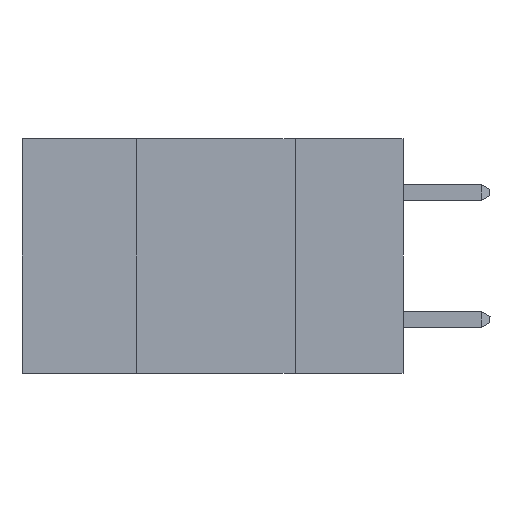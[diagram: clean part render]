
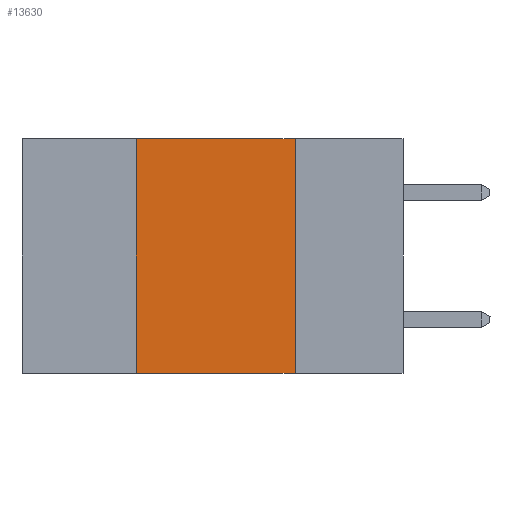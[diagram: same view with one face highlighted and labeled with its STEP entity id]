
A CAD part, left-side view. The second image highlights one B-rep face of the part: STEP entity #13630.
In plain terms, the highlighted planar face has unit normal (-1, 0, 0).
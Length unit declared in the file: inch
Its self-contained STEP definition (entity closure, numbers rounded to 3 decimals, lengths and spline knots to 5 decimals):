
#1485 = FACE_OUTER_BOUND ( 'NONE', #4667, .T. ) ;
#1644 = CARTESIAN_POINT ( 'NONE',  ( 0., 0.42, 0. ) ) ;
#1658 = CARTESIAN_POINT ( 'NONE',  ( 0., 0.6, -0.37 ) ) ;
#2081 = CARTESIAN_POINT ( 'NONE',  ( 0., 0.42, -0.37 ) ) ;
#2156 = EDGE_CURVE ( 'NONE', #14228, #9440, #12163, .T. ) ;
#3195 = VERTEX_POINT ( 'NONE', #16575 ) ;
#4179 = ORIENTED_EDGE ( 'NONE', *, *, #10590, .F. ) ;
#4345 = DIRECTION ( 'NONE',  ( 0., -1., 0. ) ) ;
#4667 = EDGE_LOOP ( 'NONE', ( #4179, #13762, #14377, #10025 ) ) ;
#5175 = DIRECTION ( 'NONE',  ( 0., 0., -1. ) ) ;
#5305 = CARTESIAN_POINT ( 'NONE',  ( 0., 0.17, 0. ) ) ;
#5422 = AXIS2_PLACEMENT_3D ( 'NONE', #14116, #6511, #5175 ) ;
#5824 = DIRECTION ( 'NONE',  ( 0., 0., 1. ) ) ;
#6511 = DIRECTION ( 'NONE',  ( 1., 0., 0. ) ) ;
#8039 = LINE ( 'NONE', #9314, #12265 ) ;
#8365 = VECTOR ( 'NONE', #5824, 39.37008 ) ;
#8670 = VERTEX_POINT ( 'NONE', #5305 ) ;
#9046 = PLANE ( 'NONE',  #5422 ) ;
#9314 = CARTESIAN_POINT ( 'NONE',  ( 0., 0.17, 0. ) ) ;
#9440 = VERTEX_POINT ( 'NONE', #13012 ) ;
#10025 = ORIENTED_EDGE ( 'NONE', *, *, #11953, .T. ) ;
#10590 = EDGE_CURVE ( 'NONE', #8670, #3195, #8039, .T. ) ;
#10997 = VECTOR ( 'NONE', #4345, 39.37008 ) ;
#11953 = EDGE_CURVE ( 'NONE', #14228, #3195, #13374, .T. ) ;
#12058 = LINE ( 'NONE', #14581, #14069 ) ;
#12094 = DIRECTION ( 'NONE',  ( 0., 0., -1. ) ) ;
#12163 = LINE ( 'NONE', #1644, #8365 ) ;
#12265 = VECTOR ( 'NONE', #12094, 39.37008 ) ;
#13012 = CARTESIAN_POINT ( 'NONE',  ( 0., 0.42, 0. ) ) ;
#13158 = DIRECTION ( 'NONE',  ( 0., -1., 0. ) ) ;
#13374 = LINE ( 'NONE', #1658, #10997 ) ;
#13630 = ADVANCED_FACE ( 'NONE', ( #1485 ), #9046, .F. ) ;
#13762 = ORIENTED_EDGE ( 'NONE', *, *, #14998, .F. ) ;
#14069 = VECTOR ( 'NONE', #13158, 39.37008 ) ;
#14116 = CARTESIAN_POINT ( 'NONE',  ( 0., 0.6, 0. ) ) ;
#14228 = VERTEX_POINT ( 'NONE', #2081 ) ;
#14377 = ORIENTED_EDGE ( 'NONE', *, *, #2156, .F. ) ;
#14581 = CARTESIAN_POINT ( 'NONE',  ( 0., 0.6, 0. ) ) ;
#14998 = EDGE_CURVE ( 'NONE', #9440, #8670, #12058, .T. ) ;
#16575 = CARTESIAN_POINT ( 'NONE',  ( 0., 0.17, -0.37 ) ) ;
